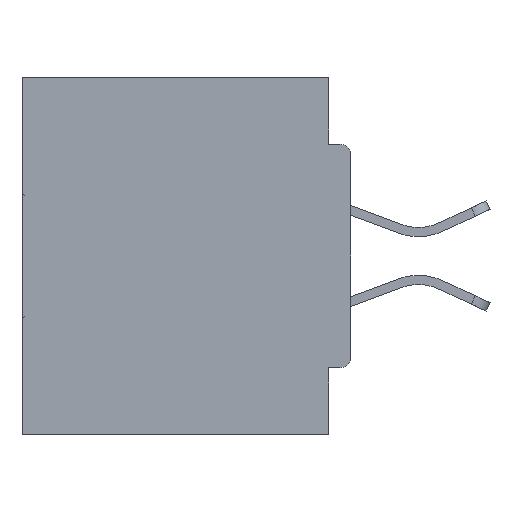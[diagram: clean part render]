
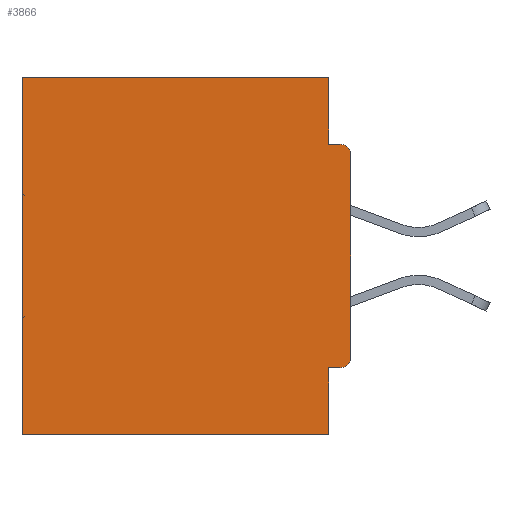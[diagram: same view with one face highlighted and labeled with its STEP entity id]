
A CAD part, left-side view. The second image highlights one B-rep face of the part: STEP entity #3866.
In plain terms, the highlighted planar face has unit normal (-1, 0, 0).
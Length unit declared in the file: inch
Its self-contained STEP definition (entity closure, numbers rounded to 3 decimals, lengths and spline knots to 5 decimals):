
#837 = VERTEX_POINT ( 'NONE', #12155 ) ;
#1059 = ORIENTED_EDGE ( 'NONE', *, *, #6574, .T. ) ;
#1071 = DIRECTION ( 'NONE',  ( 0., 1., 0. ) ) ;
#1134 = VERTEX_POINT ( 'NONE', #37885 ) ;
#1164 = LINE ( 'NONE', #37832, #29558 ) ;
#1251 = ORIENTED_EDGE ( 'NONE', *, *, #42209, .F. ) ;
#1406 = CARTESIAN_POINT ( 'NONE',  ( 0.298, 0., -0.1085 ) ) ;
#1536 = VECTOR ( 'NONE', #17095, 39.37008 ) ;
#1785 = ORIENTED_EDGE ( 'NONE', *, *, #19687, .T. ) ;
#1824 = DIRECTION ( 'NONE',  ( 0., 0., -1. ) ) ;
#1985 = VECTOR ( 'NONE', #30681, 39.37008 ) ;
#3572 = DIRECTION ( 'NONE',  ( -1., 0., 0. ) ) ;
#3866 = ADVANCED_FACE ( 'NONE', ( #37852 ), #22268, .F. ) ;
#3960 = CARTESIAN_POINT ( 'NONE',  ( 0.298, 0.46, 0. ) ) ;
#4668 = CARTESIAN_POINT ( 'NONE',  ( 0.298, 0., 0. ) ) ;
#4953 = DIRECTION ( 'NONE',  ( 1., 0., 0. ) ) ;
#6128 = AXIS2_PLACEMENT_3D ( 'NONE', #34449, #3572, #17279 ) ;
#6574 = EDGE_CURVE ( 'NONE', #1134, #30812, #18927, .T. ) ;
#6595 = VECTOR ( 'NONE', #7918, 39.37008 ) ;
#6793 = DIRECTION ( 'NONE',  ( -1., 0., 0. ) ) ;
#7182 = LINE ( 'NONE', #16057, #11451 ) ;
#7918 = DIRECTION ( 'NONE',  ( 0., -1., 0. ) ) ;
#8741 = VECTOR ( 'NONE', #1071, 39.37008 ) ;
#8811 = CARTESIAN_POINT ( 'NONE',  ( 0.298, 0.031, -0.4065 ) ) ;
#8876 = LINE ( 'NONE', #26342, #1985 ) ;
#8963 = VERTEX_POINT ( 'NONE', #21074 ) ;
#10130 = CARTESIAN_POINT ( 'NONE',  ( 0.298, 0.031, 0. ) ) ;
#10610 = CARTESIAN_POINT ( 'NONE',  ( 0.298, 0.031, -0.5 ) ) ;
#11198 = EDGE_CURVE ( 'NONE', #25279, #30812, #8876, .T. ) ;
#11251 = VERTEX_POINT ( 'NONE', #31270 ) ;
#11451 = VECTOR ( 'NONE', #19944, 39.37008 ) ;
#12155 = CARTESIAN_POINT ( 'NONE',  ( 0.298, 0.031, -0.0935 ) ) ;
#12514 = ORIENTED_EDGE ( 'NONE', *, *, #39605, .F. ) ;
#13479 = EDGE_CURVE ( 'NONE', #8963, #32832, #1164, .T. ) ;
#14143 = ORIENTED_EDGE ( 'NONE', *, *, #13479, .F. ) ;
#16057 = CARTESIAN_POINT ( 'NONE',  ( 0.298, 0.031, -0.5 ) ) ;
#16136 = VERTEX_POINT ( 'NONE', #10130 ) ;
#16948 = CARTESIAN_POINT ( 'NONE',  ( 0.298, 0.015, -0.3915 ) ) ;
#17095 = DIRECTION ( 'NONE',  ( 0., 0., -1. ) ) ;
#17279 = DIRECTION ( 'NONE',  ( 0., 0., -1. ) ) ;
#17624 = DIRECTION ( 'NONE',  ( 0., 0., -1. ) ) ;
#18038 = LINE ( 'NONE', #3960, #1536 ) ;
#18927 = CIRCLE ( 'NONE', #26759, 0.015 ) ;
#19463 = EDGE_CURVE ( 'NONE', #16136, #837, #7182, .T. ) ;
#19687 = EDGE_CURVE ( 'NONE', #25279, #11251, #25947, .T. ) ;
#19944 = DIRECTION ( 'NONE',  ( 0., 0., -1. ) ) ;
#20614 = ORIENTED_EDGE ( 'NONE', *, *, #34903, .F. ) ;
#21074 = CARTESIAN_POINT ( 'NONE',  ( 0.298, 0.031, -0.5 ) ) ;
#22268 = PLANE ( 'NONE',  #23806 ) ;
#22387 = EDGE_LOOP ( 'NONE', ( #1785, #1251, #27278, #39643, #26312, #14143, #20614, #12514, #1059, #29911 ) ) ;
#23236 = CARTESIAN_POINT ( 'NONE',  ( 0.298, 0.46, -0.5 ) ) ;
#23707 = VERTEX_POINT ( 'NONE', #25593 ) ;
#23806 = AXIS2_PLACEMENT_3D ( 'NONE', #32203, #4953, #1824 ) ;
#23825 = VERTEX_POINT ( 'NONE', #8811 ) ;
#25279 = VERTEX_POINT ( 'NONE', #1406 ) ;
#25593 = CARTESIAN_POINT ( 'NONE',  ( 0.298, 0.46, 0. ) ) ;
#25947 = CIRCLE ( 'NONE', #6128, 0.015 ) ;
#26181 = CARTESIAN_POINT ( 'NONE',  ( 0.298, 0., -0.3915 ) ) ;
#26312 = ORIENTED_EDGE ( 'NONE', *, *, #34362, .T. ) ;
#26342 = CARTESIAN_POINT ( 'NONE',  ( 0.298, 0., 0. ) ) ;
#26759 = AXIS2_PLACEMENT_3D ( 'NONE', #16948, #6793, #34245 ) ;
#27278 = ORIENTED_EDGE ( 'NONE', *, *, #19463, .F. ) ;
#29130 = LINE ( 'NONE', #4668, #8741 ) ;
#29558 = VECTOR ( 'NONE', #40989, 39.37008 ) ;
#29911 = ORIENTED_EDGE ( 'NONE', *, *, #11198, .F. ) ;
#30681 = DIRECTION ( 'NONE',  ( 0., 0., -1. ) ) ;
#30812 = VERTEX_POINT ( 'NONE', #26181 ) ;
#31270 = CARTESIAN_POINT ( 'NONE',  ( 0.298, 0.015, -0.0935 ) ) ;
#31901 = CARTESIAN_POINT ( 'NONE',  ( 0.298, 0., -0.0935 ) ) ;
#32203 = CARTESIAN_POINT ( 'NONE',  ( 0.298, 0., 0. ) ) ;
#32787 = CARTESIAN_POINT ( 'NONE',  ( 0.298, 0., -0.4065 ) ) ;
#32832 = VERTEX_POINT ( 'NONE', #23236 ) ;
#34245 = DIRECTION ( 'NONE',  ( 0., 0., -1. ) ) ;
#34362 = EDGE_CURVE ( 'NONE', #23707, #32832, #18038, .T. ) ;
#34449 = CARTESIAN_POINT ( 'NONE',  ( 0.298, 0.015, -0.1085 ) ) ;
#34673 = VECTOR ( 'NONE', #17624, 39.37008 ) ;
#34903 = EDGE_CURVE ( 'NONE', #23825, #8963, #43323, .T. ) ;
#35824 = LINE ( 'NONE', #32787, #40127 ) ;
#37832 = CARTESIAN_POINT ( 'NONE',  ( 0.298, 0., -0.5 ) ) ;
#37852 = FACE_OUTER_BOUND ( 'NONE', #22387, .T. ) ;
#37885 = CARTESIAN_POINT ( 'NONE',  ( 0.298, 0.015, -0.4065 ) ) ;
#38280 = LINE ( 'NONE', #31901, #6595 ) ;
#39605 = EDGE_CURVE ( 'NONE', #1134, #23825, #35824, .T. ) ;
#39643 = ORIENTED_EDGE ( 'NONE', *, *, #42254, .T. ) ;
#39729 = DIRECTION ( 'NONE',  ( 0., 1., 0. ) ) ;
#40127 = VECTOR ( 'NONE', #39729, 39.37008 ) ;
#40989 = DIRECTION ( 'NONE',  ( 0., 1., 0. ) ) ;
#42209 = EDGE_CURVE ( 'NONE', #837, #11251, #38280, .T. ) ;
#42254 = EDGE_CURVE ( 'NONE', #16136, #23707, #29130, .T. ) ;
#43323 = LINE ( 'NONE', #10610, #34673 ) ;
